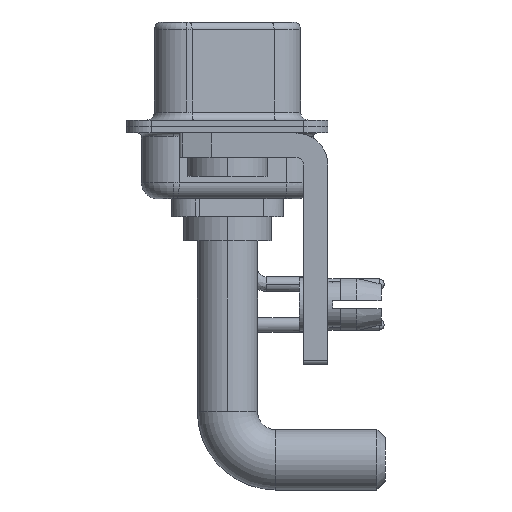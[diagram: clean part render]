
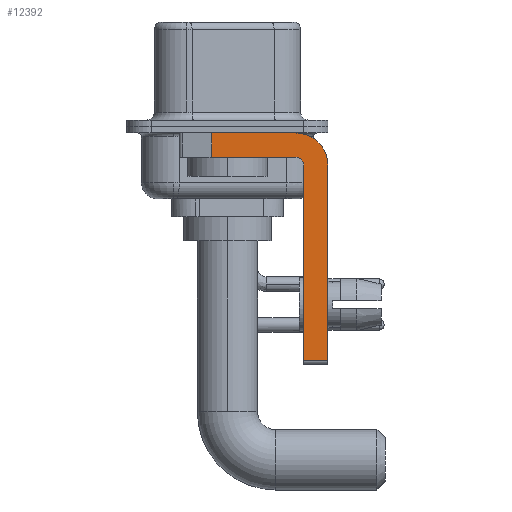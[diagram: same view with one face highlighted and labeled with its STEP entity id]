
A CAD part, left-side view. The second image highlights one B-rep face of the part: STEP entity #12392.
In plain terms, the highlighted planar face has unit normal (-1, 0, 0).
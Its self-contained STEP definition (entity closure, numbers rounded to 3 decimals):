
#864 = AXIS2_PLACEMENT_3D ( 'NONE', #25892, #1831, #4320 ) ;
#1646 = VECTOR ( 'NONE', #18142, 1000. ) ;
#1831 = DIRECTION ( 'NONE',  ( 1., 0., 0. ) ) ;
#2648 = CIRCLE ( 'NONE', #27779, 2. ) ;
#3179 = EDGE_CURVE ( 'NONE', #6799, #27380, #3791, .T. ) ;
#3377 = CARTESIAN_POINT ( 'NONE',  ( -2.9, -4.75, -2.4 ) ) ;
#3791 = LINE ( 'NONE', #20330, #5761 ) ;
#3815 = CARTESIAN_POINT ( 'NONE',  ( -2.9, 3., -0.4 ) ) ;
#3910 = ORIENTED_EDGE ( 'NONE', *, *, #3179, .F. ) ;
#4141 = EDGE_CURVE ( 'NONE', #9738, #10826, #7298, .T. ) ;
#4320 = DIRECTION ( 'NONE',  ( 0., 0., -1. ) ) ;
#5048 = LINE ( 'NONE', #15148, #12135 ) ;
#5214 = VERTEX_POINT ( 'NONE', #8999 ) ;
#5761 = VECTOR ( 'NONE', #27717, 1000. ) ;
#6042 = DIRECTION ( 'NONE',  ( 0., 0., -1. ) ) ;
#6799 = VERTEX_POINT ( 'NONE', #13939 ) ;
#7246 = DIRECTION ( 'NONE',  ( 0., 1., 0. ) ) ;
#7298 = CIRCLE ( 'NONE', #20880, 0.5 ) ;
#7774 = DIRECTION ( 'NONE',  ( 0., 0., 1. ) ) ;
#8044 = VECTOR ( 'NONE', #20285, 1000. ) ;
#8321 = ORIENTED_EDGE ( 'NONE', *, *, #19393, .F. ) ;
#8463 = LINE ( 'NONE', #30351, #8044 ) ;
#8701 = CARTESIAN_POINT ( 'NONE',  ( -2.9, -4.25, -2.4 ) ) ;
#8999 = CARTESIAN_POINT ( 'NONE',  ( -2.9, 0.978, -1.9 ) ) ;
#9062 = DIRECTION ( 'NONE',  ( 0., 0., -1. ) ) ;
#9738 = VERTEX_POINT ( 'NONE', #3377 ) ;
#9754 = EDGE_CURVE ( 'NONE', #22746, #5214, #22580, .T. ) ;
#10826 = VERTEX_POINT ( 'NONE', #14468 ) ;
#11583 = CARTESIAN_POINT ( 'NONE',  ( -2.9, -4.25, -0.4 ) ) ;
#11839 = ORIENTED_EDGE ( 'NONE', *, *, #17887, .F. ) ;
#11868 = ORIENTED_EDGE ( 'NONE', *, *, #9754, .T. ) ;
#11896 = LINE ( 'NONE', #19277, #27050 ) ;
#12135 = VECTOR ( 'NONE', #7246, 1000. ) ;
#12392 = ADVANCED_FACE ( 'NONE', ( #23374 ), #25596, .F. ) ;
#12494 = CARTESIAN_POINT ( 'NONE',  ( -2.9, 0.978, -0.4 ) ) ;
#12671 = CARTESIAN_POINT ( 'NONE',  ( -2.9, 0.978, -1.9 ) ) ;
#13118 = LINE ( 'NONE', #3815, #1646 ) ;
#13559 = EDGE_CURVE ( 'NONE', #20102, #9738, #11896, .T. ) ;
#13939 = CARTESIAN_POINT ( 'NONE',  ( -2.9, -6.25, -2.4 ) ) ;
#14468 = CARTESIAN_POINT ( 'NONE',  ( -2.9, -4.25, -1.9 ) ) ;
#15148 = CARTESIAN_POINT ( 'NONE',  ( -2.9, -4.25, -1.9 ) ) ;
#15553 = VERTEX_POINT ( 'NONE', #11583 ) ;
#15608 = ORIENTED_EDGE ( 'NONE', *, *, #4141, .F. ) ;
#17591 = CARTESIAN_POINT ( 'NONE',  ( -2.9, -6.25, -14.55 ) ) ;
#17887 = EDGE_CURVE ( 'NONE', #10826, #5214, #5048, .T. ) ;
#18142 = DIRECTION ( 'NONE',  ( 0., -1., 0. ) ) ;
#18621 = DIRECTION ( 'NONE',  ( -1., 0., 0. ) ) ;
#19277 = CARTESIAN_POINT ( 'NONE',  ( -2.9, -4.75, -14.8 ) ) ;
#19393 = EDGE_CURVE ( 'NONE', #15553, #6799, #2648, .T. ) ;
#20011 = CARTESIAN_POINT ( 'NONE',  ( -2.9, -4.75, -14.55 ) ) ;
#20102 = VERTEX_POINT ( 'NONE', #20011 ) ;
#20285 = DIRECTION ( 'NONE',  ( 0., -1., 0. ) ) ;
#20330 = CARTESIAN_POINT ( 'NONE',  ( -2.9, -6.25, -2.4 ) ) ;
#20880 = AXIS2_PLACEMENT_3D ( 'NONE', #8701, #18621, #27761 ) ;
#21642 = EDGE_CURVE ( 'NONE', #22746, #15553, #13118, .T. ) ;
#21813 = CARTESIAN_POINT ( 'NONE',  ( -2.9, -4.25, -2.4 ) ) ;
#22580 = LINE ( 'NONE', #12671, #29464 ) ;
#22746 = VERTEX_POINT ( 'NONE', #12494 ) ;
#23360 = ORIENTED_EDGE ( 'NONE', *, *, #30221, .T. ) ;
#23374 = FACE_OUTER_BOUND ( 'NONE', #28636, .T. ) ;
#24520 = ORIENTED_EDGE ( 'NONE', *, *, #21642, .F. ) ;
#25596 = PLANE ( 'NONE',  #864 ) ;
#25892 = CARTESIAN_POINT ( 'NONE',  ( -2.9, -4.25, -2.4 ) ) ;
#27050 = VECTOR ( 'NONE', #7774, 1000. ) ;
#27380 = VERTEX_POINT ( 'NONE', #17591 ) ;
#27717 = DIRECTION ( 'NONE',  ( 0., 0., -1. ) ) ;
#27761 = DIRECTION ( 'NONE',  ( 0., 0., 1. ) ) ;
#27779 = AXIS2_PLACEMENT_3D ( 'NONE', #21813, #28282, #9062 ) ;
#27827 = ORIENTED_EDGE ( 'NONE', *, *, #13559, .F. ) ;
#28282 = DIRECTION ( 'NONE',  ( 1., 0., 0. ) ) ;
#28636 = EDGE_LOOP ( 'NONE', ( #24520, #11868, #11839, #15608, #27827, #23360, #3910, #8321 ) ) ;
#29464 = VECTOR ( 'NONE', #6042, 1000. ) ;
#30221 = EDGE_CURVE ( 'NONE', #20102, #27380, #8463, .T. ) ;
#30351 = CARTESIAN_POINT ( 'NONE',  ( -2.9, -4.25, -14.55 ) ) ;
